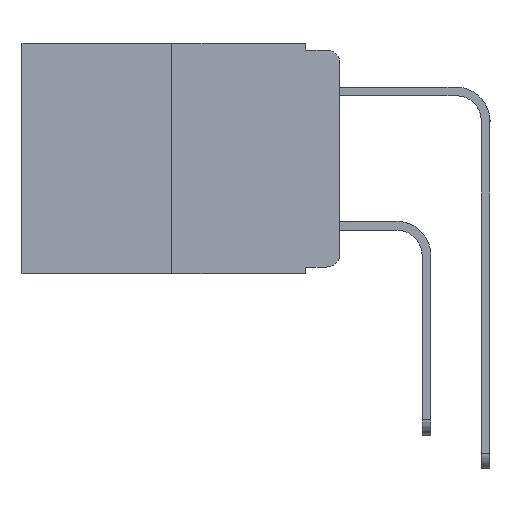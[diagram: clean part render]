
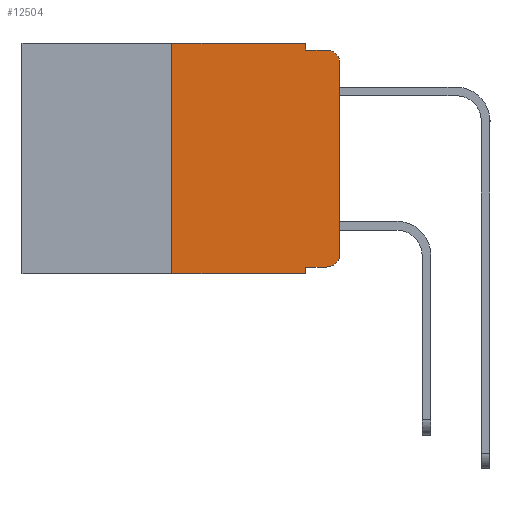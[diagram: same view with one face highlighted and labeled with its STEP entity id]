
A CAD part, left-side view. The second image highlights one B-rep face of the part: STEP entity #12504.
In plain terms, the highlighted planar face has unit normal (-1, 0, 0).
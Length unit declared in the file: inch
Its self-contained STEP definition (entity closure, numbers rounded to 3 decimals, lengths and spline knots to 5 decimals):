
#136 = CARTESIAN_POINT ( 'NONE',  ( 0., 0.051, 0. ) ) ;
#435 = DIRECTION ( 'NONE',  ( 0., 0., -1. ) ) ;
#448 = VERTEX_POINT ( 'NONE', #10867 ) ;
#805 = CARTESIAN_POINT ( 'NONE',  ( 0., 0.02, -0.03 ) ) ;
#826 = CARTESIAN_POINT ( 'NONE',  ( 0., 0.25, 0. ) ) ;
#899 = DIRECTION ( 'NONE',  ( -1., 0., 0. ) ) ;
#1271 = DIRECTION ( 'NONE',  ( 0., 0., -1. ) ) ;
#1530 = LINE ( 'NONE', #136, #2041 ) ;
#1844 = DIRECTION ( 'NONE',  ( 0., 0., -1. ) ) ;
#2041 = VECTOR ( 'NONE', #1844, 39.37008 ) ;
#2299 = LINE ( 'NONE', #18637, #18957 ) ;
#2964 = EDGE_CURVE ( 'NONE', #10681, #16437, #2299, .T. ) ;
#3165 = CARTESIAN_POINT ( 'NONE',  ( 0., 0.051, 0. ) ) ;
#3192 = VERTEX_POINT ( 'NONE', #16756 ) ;
#3298 = FACE_OUTER_BOUND ( 'NONE', #17430, .T. ) ;
#3475 = ORIENTED_EDGE ( 'NONE', *, *, #5322, .T. ) ;
#3626 = CARTESIAN_POINT ( 'NONE',  ( 0., 0.051, -0.01 ) ) ;
#3755 = CARTESIAN_POINT ( 'NONE',  ( 0., 0.473, 0. ) ) ;
#4407 = CARTESIAN_POINT ( 'NONE',  ( 0., 0.02, -0.333 ) ) ;
#4423 = VECTOR ( 'NONE', #5908, 39.37008 ) ;
#4499 = CARTESIAN_POINT ( 'NONE',  ( 0., 0.051, -0.343 ) ) ;
#5255 = EDGE_CURVE ( 'NONE', #18740, #12425, #6535, .T. ) ;
#5322 = EDGE_CURVE ( 'NONE', #10655, #448, #9458, .T. ) ;
#5336 = DIRECTION ( 'NONE',  ( 0., -1., 0. ) ) ;
#5908 = DIRECTION ( 'NONE',  ( 0., 0., 1. ) ) ;
#6358 = DIRECTION ( 'NONE',  ( 0., -1., 0. ) ) ;
#6535 = LINE ( 'NONE', #3755, #14724 ) ;
#6695 = ORIENTED_EDGE ( 'NONE', *, *, #16332, .T. ) ;
#7359 = ORIENTED_EDGE ( 'NONE', *, *, #14138, .F. ) ;
#7381 = CARTESIAN_POINT ( 'NONE',  ( 0., 0.25, 0. ) ) ;
#7510 = AXIS2_PLACEMENT_3D ( 'NONE', #805, #899, #1271 ) ;
#8508 = CARTESIAN_POINT ( 'NONE',  ( 0., 0.02, -0.313 ) ) ;
#8714 = CARTESIAN_POINT ( 'NONE',  ( 0., 0.473, 0. ) ) ;
#9088 = VERTEX_POINT ( 'NONE', #16570 ) ;
#9421 = VERTEX_POINT ( 'NONE', #4407 ) ;
#9441 = DIRECTION ( 'NONE',  ( 0., -1., 0. ) ) ;
#9458 = CIRCLE ( 'NONE', #7510, 0.02 ) ;
#9484 = ORIENTED_EDGE ( 'NONE', *, *, #20388, .F. ) ;
#9491 = LINE ( 'NONE', #20441, #17454 ) ;
#9573 = ORIENTED_EDGE ( 'NONE', *, *, #19364, .F. ) ;
#9779 = DIRECTION ( 'NONE',  ( 0., 0., -1. ) ) ;
#9839 = ORIENTED_EDGE ( 'NONE', *, *, #5255, .F. ) ;
#9854 = ORIENTED_EDGE ( 'NONE', *, *, #17937, .T. ) ;
#9937 = VECTOR ( 'NONE', #9779, 39.37008 ) ;
#9980 = ORIENTED_EDGE ( 'NONE', *, *, #2964, .T. ) ;
#10010 = ORIENTED_EDGE ( 'NONE', *, *, #12379, .F. ) ;
#10170 = DIRECTION ( 'NONE',  ( 0., 0., -1. ) ) ;
#10274 = AXIS2_PLACEMENT_3D ( 'NONE', #8508, #19611, #10170 ) ;
#10320 = CIRCLE ( 'NONE', #10274, 0.02 ) ;
#10347 = CARTESIAN_POINT ( 'NONE',  ( 0., 0.25, -0.343 ) ) ;
#10353 = DIRECTION ( 'NONE',  ( 1., 0., 0. ) ) ;
#10407 = DIRECTION ( 'NONE',  ( 0., -1., 0. ) ) ;
#10447 = VERTEX_POINT ( 'NONE', #3626 ) ;
#10655 = VERTEX_POINT ( 'NONE', #13506 ) ;
#10681 = VERTEX_POINT ( 'NONE', #10347 ) ;
#10867 = CARTESIAN_POINT ( 'NONE',  ( 0., 0.02, -0.01 ) ) ;
#11155 = ORIENTED_EDGE ( 'NONE', *, *, #11875, .T. ) ;
#11875 = EDGE_CURVE ( 'NONE', #9421, #9088, #10320, .T. ) ;
#12379 = EDGE_CURVE ( 'NONE', #3192, #16437, #1530, .T. ) ;
#12425 = VERTEX_POINT ( 'NONE', #16549 ) ;
#12504 = ADVANCED_FACE ( 'NONE', ( #3298 ), #18226, .F. ) ;
#13506 = CARTESIAN_POINT ( 'NONE',  ( 0., 0., -0.03 ) ) ;
#13685 = LINE ( 'NONE', #3165, #9937 ) ;
#14138 = EDGE_CURVE ( 'NONE', #10447, #448, #9491, .T. ) ;
#14724 = VECTOR ( 'NONE', #6358, 39.37008 ) ;
#14884 = LINE ( 'NONE', #7381, #18524 ) ;
#15067 = LINE ( 'NONE', #15137, #19213 ) ;
#15137 = CARTESIAN_POINT ( 'NONE',  ( 0., 0.051, -0.333 ) ) ;
#15685 = CARTESIAN_POINT ( 'NONE',  ( 0., 0., 0. ) ) ;
#15876 = AXIS2_PLACEMENT_3D ( 'NONE', #8714, #10353, #435 ) ;
#16332 = EDGE_CURVE ( 'NONE', #9088, #10655, #16866, .T. ) ;
#16437 = VERTEX_POINT ( 'NONE', #4499 ) ;
#16549 = CARTESIAN_POINT ( 'NONE',  ( 0., 0.051, 0. ) ) ;
#16570 = CARTESIAN_POINT ( 'NONE',  ( 0., 0., -0.313 ) ) ;
#16756 = CARTESIAN_POINT ( 'NONE',  ( 0., 0.051, -0.333 ) ) ;
#16866 = LINE ( 'NONE', #15685, #4423 ) ;
#17430 = EDGE_LOOP ( 'NONE', ( #6695, #3475, #7359, #9573, #9839, #9484, #9980, #10010, #9854, #11155 ) ) ;
#17454 = VECTOR ( 'NONE', #9441, 39.37008 ) ;
#17937 = EDGE_CURVE ( 'NONE', #3192, #9421, #15067, .T. ) ;
#18226 = PLANE ( 'NONE',  #15876 ) ;
#18524 = VECTOR ( 'NONE', #20137, 39.37008 ) ;
#18637 = CARTESIAN_POINT ( 'NONE',  ( 0., 0.473, -0.343 ) ) ;
#18740 = VERTEX_POINT ( 'NONE', #826 ) ;
#18957 = VECTOR ( 'NONE', #10407, 39.37008 ) ;
#19213 = VECTOR ( 'NONE', #5336, 39.37008 ) ;
#19364 = EDGE_CURVE ( 'NONE', #12425, #10447, #13685, .T. ) ;
#19611 = DIRECTION ( 'NONE',  ( -1., 0., 0. ) ) ;
#20137 = DIRECTION ( 'NONE',  ( 0., 0., 1. ) ) ;
#20388 = EDGE_CURVE ( 'NONE', #10681, #18740, #14884, .T. ) ;
#20441 = CARTESIAN_POINT ( 'NONE',  ( 0., 0.051, -0.01 ) ) ;
